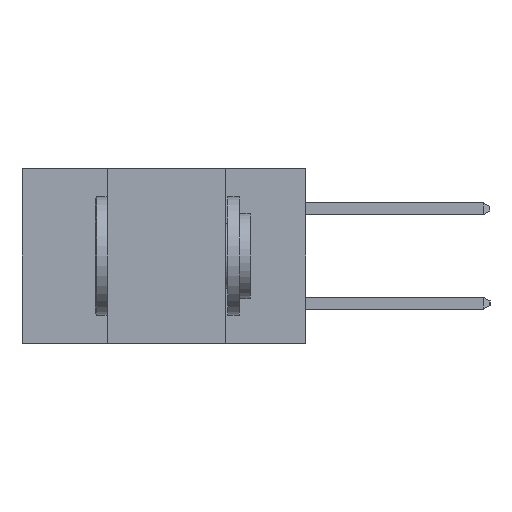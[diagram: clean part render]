
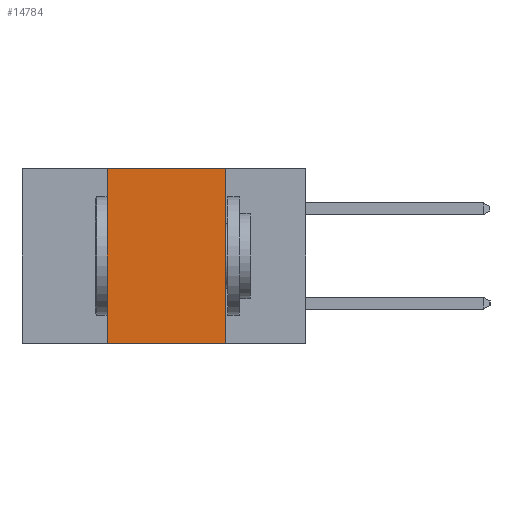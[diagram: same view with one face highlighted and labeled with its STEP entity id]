
A CAD part, left-side view. The second image highlights one B-rep face of the part: STEP entity #14784.
In plain terms, the highlighted planar face has unit normal (-1, 0, 0).
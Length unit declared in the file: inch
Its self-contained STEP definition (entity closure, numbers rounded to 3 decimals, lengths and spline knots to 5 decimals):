
#120 = LINE ( 'NONE', #15031, #11677 ) ;
#838 = LINE ( 'NONE', #7542, #11727 ) ;
#2783 = DIRECTION ( 'NONE',  ( 0., -1., 0. ) ) ;
#3175 = ORIENTED_EDGE ( 'NONE', *, *, #26059, .F. ) ;
#3224 = CARTESIAN_POINT ( 'NONE',  ( 0., 0.42, -0.37 ) ) ;
#3426 = VECTOR ( 'NONE', #24068, 39.37008 ) ;
#3999 = CARTESIAN_POINT ( 'NONE',  ( 0., 0.6, 0. ) ) ;
#4880 = LINE ( 'NONE', #12518, #25783 ) ;
#5811 = VERTEX_POINT ( 'NONE', #3224 ) ;
#6025 = DIRECTION ( 'NONE',  ( 1., 0., 0. ) ) ;
#6207 = CARTESIAN_POINT ( 'NONE',  ( 0., 0.17, -0.37 ) ) ;
#7542 = CARTESIAN_POINT ( 'NONE',  ( 0., 0.42, -0.37 ) ) ;
#7861 = CARTESIAN_POINT ( 'NONE',  ( 0., 0.6, 0. ) ) ;
#8527 = EDGE_LOOP ( 'NONE', ( #23498, #3175, #8606, #25369 ) ) ;
#8606 = ORIENTED_EDGE ( 'NONE', *, *, #25218, .F. ) ;
#9411 = EDGE_CURVE ( 'NONE', #5811, #14875, #120, .T. ) ;
#11401 = VERTEX_POINT ( 'NONE', #17930 ) ;
#11677 = VECTOR ( 'NONE', #2783, 39.37008 ) ;
#11727 = VECTOR ( 'NONE', #13739, 39.37008 ) ;
#12518 = CARTESIAN_POINT ( 'NONE',  ( 0., 0.17, -0.37 ) ) ;
#12616 = CARTESIAN_POINT ( 'NONE',  ( 0., 0.17, 0. ) ) ;
#13739 = DIRECTION ( 'NONE',  ( 0., 0., 1. ) ) ;
#14784 = ADVANCED_FACE ( 'NONE', ( #22311 ), #16237, .F. ) ;
#14875 = VERTEX_POINT ( 'NONE', #6207 ) ;
#15031 = CARTESIAN_POINT ( 'NONE',  ( 0., 0.6, -0.37 ) ) ;
#15635 = VERTEX_POINT ( 'NONE', #12616 ) ;
#16237 = PLANE ( 'NONE',  #16935 ) ;
#16713 = DIRECTION ( 'NONE',  ( 0., 0., -1. ) ) ;
#16935 = AXIS2_PLACEMENT_3D ( 'NONE', #3999, #6025, #20327 ) ;
#17930 = CARTESIAN_POINT ( 'NONE',  ( 0., 0.42, 0. ) ) ;
#19692 = LINE ( 'NONE', #7861, #3426 ) ;
#20327 = DIRECTION ( 'NONE',  ( 0., 0., -1. ) ) ;
#22046 = EDGE_CURVE ( 'NONE', #15635, #14875, #4880, .T. ) ;
#22311 = FACE_OUTER_BOUND ( 'NONE', #8527, .T. ) ;
#23498 = ORIENTED_EDGE ( 'NONE', *, *, #22046, .F. ) ;
#24068 = DIRECTION ( 'NONE',  ( 0., -1., 0. ) ) ;
#25218 = EDGE_CURVE ( 'NONE', #5811, #11401, #838, .T. ) ;
#25369 = ORIENTED_EDGE ( 'NONE', *, *, #9411, .T. ) ;
#25783 = VECTOR ( 'NONE', #16713, 39.37008 ) ;
#26059 = EDGE_CURVE ( 'NONE', #11401, #15635, #19692, .T. ) ;
